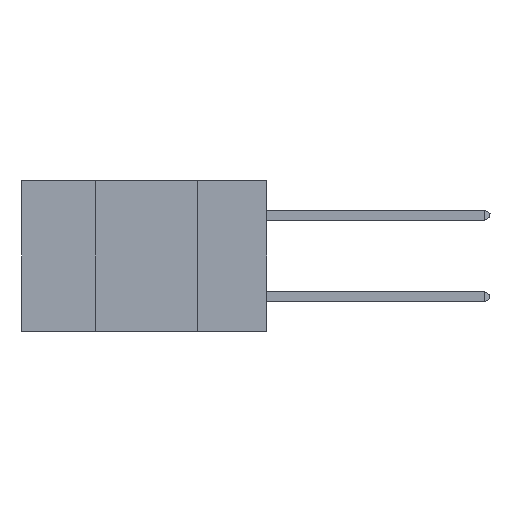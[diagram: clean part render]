
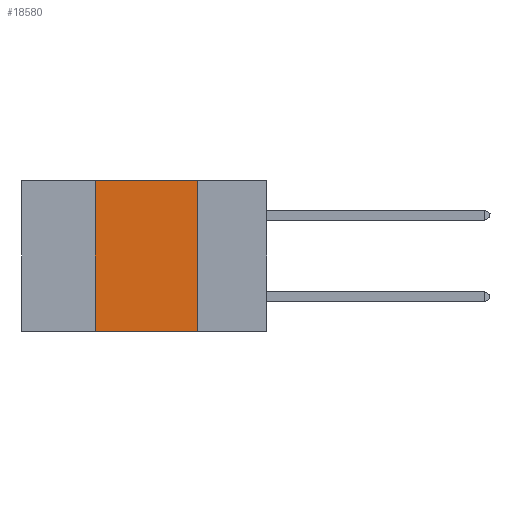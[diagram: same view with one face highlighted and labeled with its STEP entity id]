
A CAD part, left-side view. The second image highlights one B-rep face of the part: STEP entity #18580.
In plain terms, the highlighted planar face has unit normal (-1, 0, 0).
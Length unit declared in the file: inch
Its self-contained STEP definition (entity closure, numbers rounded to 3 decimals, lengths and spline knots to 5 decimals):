
#325 = VECTOR ( 'NONE', #17294, 39.37008 ) ;
#2560 = CARTESIAN_POINT ( 'NONE',  ( 0., 0.17, -0.37 ) ) ;
#3509 = DIRECTION ( 'NONE',  ( 1., 0., 0. ) ) ;
#3608 = LINE ( 'NONE', #18725, #325 ) ;
#5023 = FACE_OUTER_BOUND ( 'NONE', #9188, .T. ) ;
#5458 = CARTESIAN_POINT ( 'NONE',  ( 0., 0.17, 0. ) ) ;
#6008 = VERTEX_POINT ( 'NONE', #9640 ) ;
#6442 = DIRECTION ( 'NONE',  ( 0., 0., -1. ) ) ;
#6475 = DIRECTION ( 'NONE',  ( 0., -1., 0. ) ) ;
#6872 = LINE ( 'NONE', #14220, #13012 ) ;
#7583 = VERTEX_POINT ( 'NONE', #9025 ) ;
#8026 = AXIS2_PLACEMENT_3D ( 'NONE', #9755, #3509, #6442 ) ;
#8066 = LINE ( 'NONE', #14599, #15010 ) ;
#8319 = CARTESIAN_POINT ( 'NONE',  ( 0., 0.42, -0.37 ) ) ;
#8636 = ORIENTED_EDGE ( 'NONE', *, *, #15665, .F. ) ;
#9025 = CARTESIAN_POINT ( 'NONE',  ( 0., 0.42, 0. ) ) ;
#9188 = EDGE_LOOP ( 'NONE', ( #13210, #13788, #8636, #16199 ) ) ;
#9640 = CARTESIAN_POINT ( 'NONE',  ( 0., 0.17, 0. ) ) ;
#9755 = CARTESIAN_POINT ( 'NONE',  ( 0., 0.6, 0. ) ) ;
#11170 = VERTEX_POINT ( 'NONE', #2560 ) ;
#11404 = EDGE_CURVE ( 'NONE', #19155, #11170, #6872, .T. ) ;
#12840 = EDGE_CURVE ( 'NONE', #6008, #11170, #13013, .T. ) ;
#13012 = VECTOR ( 'NONE', #6475, 39.37008 ) ;
#13013 = LINE ( 'NONE', #5458, #13977 ) ;
#13210 = ORIENTED_EDGE ( 'NONE', *, *, #12840, .F. ) ;
#13788 = ORIENTED_EDGE ( 'NONE', *, *, #18573, .F. ) ;
#13977 = VECTOR ( 'NONE', #15743, 39.37008 ) ;
#14220 = CARTESIAN_POINT ( 'NONE',  ( 0., 0.6, -0.37 ) ) ;
#14599 = CARTESIAN_POINT ( 'NONE',  ( 0., 0.42, 0. ) ) ;
#15010 = VECTOR ( 'NONE', #17320, 39.37008 ) ;
#15665 = EDGE_CURVE ( 'NONE', #19155, #7583, #8066, .T. ) ;
#15743 = DIRECTION ( 'NONE',  ( 0., 0., -1. ) ) ;
#16199 = ORIENTED_EDGE ( 'NONE', *, *, #11404, .T. ) ;
#17294 = DIRECTION ( 'NONE',  ( 0., -1., 0. ) ) ;
#17320 = DIRECTION ( 'NONE',  ( 0., 0., 1. ) ) ;
#18573 = EDGE_CURVE ( 'NONE', #7583, #6008, #3608, .T. ) ;
#18580 = ADVANCED_FACE ( 'NONE', ( #5023 ), #18819, .F. ) ;
#18725 = CARTESIAN_POINT ( 'NONE',  ( 0., 0.6, 0. ) ) ;
#18819 = PLANE ( 'NONE',  #8026 ) ;
#19155 = VERTEX_POINT ( 'NONE', #8319 ) ;
